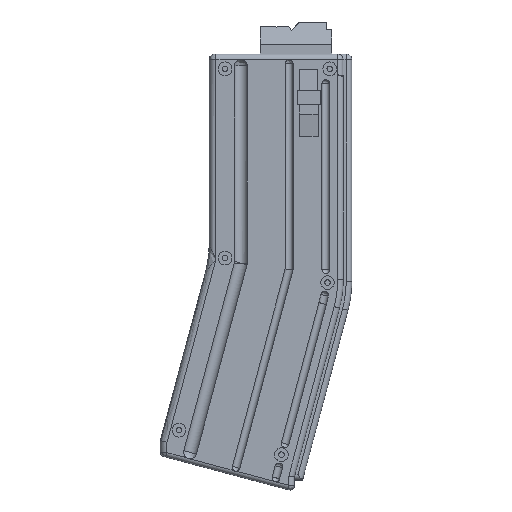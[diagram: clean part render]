
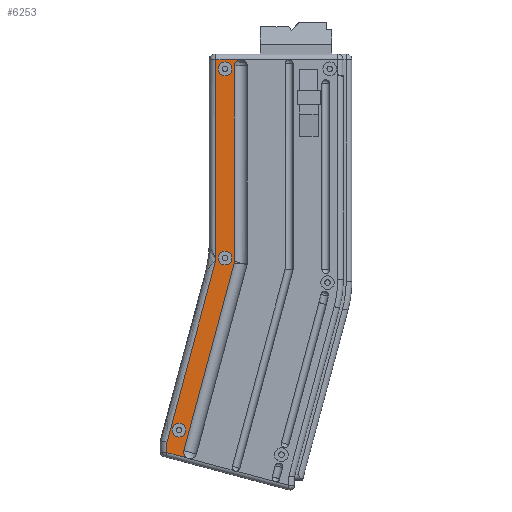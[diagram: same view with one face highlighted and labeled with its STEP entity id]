
A CAD part, front view. The second image highlights one B-rep face of the part: STEP entity #6253.
In plain terms, the highlighted planar face has unit normal (0, -1, 0).
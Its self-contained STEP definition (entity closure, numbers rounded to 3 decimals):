
#37=FACE_BOUND('',#1269,.T.);
#38=FACE_BOUND('',#1270,.T.);
#39=FACE_BOUND('',#1271,.T.);
#191=B_SPLINE_CURVE_WITH_KNOTS('',3,(#9843,#9844,#9845,#9846,#9847,#9848,
#9849,#9850,#9851,#9852,#9853,#9854),.UNSPECIFIED.,.F.,.F.,(4,2,2,2,2,4),
(0.,0.112,0.224,0.335,0.439,
0.44),.UNSPECIFIED.);
#193=B_SPLINE_CURVE_WITH_KNOTS('',3,(#9987,#9988,#9989,#9990,#9991,#9992,
#9993,#9994,#9995,#9996,#9997,#9998),.UNSPECIFIED.,.F.,.F.,(4,2,2,2,2,4),
(-0.001,0.,0.105,0.216,0.327,
0.439),.UNSPECIFIED.);
#195=B_SPLINE_CURVE_WITH_KNOTS('',3,(#10056,#10057,#10058,#10059,#10060,
#10061,#10062,#10063,#10064,#10065,#10066,#10067,#10068),.UNSPECIFIED.,
 .F.,.F.,(4,3,3,3,4),(0.,0.024,0.037,0.061,
0.073),.UNSPECIFIED.);
#656=CIRCLE('',#6703,3.075);
#657=CIRCLE('',#6704,3.075);
#658=CIRCLE('',#6705,3.075);
#876=FACE_OUTER_BOUND('',#1268,.T.);
#1268=EDGE_LOOP('',(#4353,#4354,#4355,#4356,#4357,#4358,#4359,#4360,#4361,
#4362,#4363));
#1269=EDGE_LOOP('',(#4364));
#1270=EDGE_LOOP('',(#4365));
#1271=EDGE_LOOP('',(#4366));
#1661=LINE('',#9527,#2093);
#1685=LINE('',#9873,#2117);
#1687=LINE('',#10013,#2119);
#1688=LINE('',#10071,#2120);
#1689=LINE('',#10073,#2121);
#1690=LINE('',#10075,#2122);
#1691=LINE('',#10077,#2123);
#1692=LINE('',#10078,#2124);
#2093=VECTOR('',#7355,10.);
#2117=VECTOR('',#7413,10.);
#2119=VECTOR('',#7417,10.);
#2120=VECTOR('',#7424,10.);
#2121=VECTOR('',#7425,10.);
#2122=VECTOR('',#7426,10.);
#2123=VECTOR('',#7427,10.);
#2124=VECTOR('',#7428,10.);
#2559=VERTEX_POINT('',#9524);
#2560=VERTEX_POINT('',#9526);
#2594=VERTEX_POINT('',#9842);
#2596=VERTEX_POINT('',#9871);
#2597=VERTEX_POINT('',#9984);
#2598=VERTEX_POINT('',#9986);
#2599=VERTEX_POINT('',#10012);
#2600=VERTEX_POINT('',#10070);
#2601=VERTEX_POINT('',#10072);
#2602=VERTEX_POINT('',#10074);
#2603=VERTEX_POINT('',#10076);
#2604=VERTEX_POINT('',#10079);
#2605=VERTEX_POINT('',#10081);
#2606=VERTEX_POINT('',#10083);
#3208=EDGE_CURVE('',#2559,#2560,#1661,.T.);
#3249=EDGE_CURVE('',#2559,#2594,#191,.F.);
#3253=EDGE_CURVE('',#2594,#2596,#1685,.T.);
#3255=EDGE_CURVE('',#2597,#2598,#193,.T.);
#3257=EDGE_CURVE('',#2599,#2598,#1687,.T.);
#3260=EDGE_CURVE('',#2599,#2596,#195,.T.);
#3261=EDGE_CURVE('',#2600,#2597,#1688,.T.);
#3262=EDGE_CURVE('',#2601,#2600,#1689,.T.);
#3263=EDGE_CURVE('',#2601,#2602,#1690,.T.);
#3264=EDGE_CURVE('',#2603,#2602,#1691,.T.);
#3265=EDGE_CURVE('',#2560,#2603,#1692,.T.);
#3266=EDGE_CURVE('',#2604,#2604,#656,.T.);
#3267=EDGE_CURVE('',#2605,#2605,#657,.T.);
#3268=EDGE_CURVE('',#2606,#2606,#658,.T.);
#4353=ORIENTED_EDGE('',*,*,#3260,.F.);
#4354=ORIENTED_EDGE('',*,*,#3257,.T.);
#4355=ORIENTED_EDGE('',*,*,#3255,.F.);
#4356=ORIENTED_EDGE('',*,*,#3261,.F.);
#4357=ORIENTED_EDGE('',*,*,#3262,.F.);
#4358=ORIENTED_EDGE('',*,*,#3263,.T.);
#4359=ORIENTED_EDGE('',*,*,#3264,.F.);
#4360=ORIENTED_EDGE('',*,*,#3265,.F.);
#4361=ORIENTED_EDGE('',*,*,#3208,.F.);
#4362=ORIENTED_EDGE('',*,*,#3249,.T.);
#4363=ORIENTED_EDGE('',*,*,#3253,.T.);
#4364=ORIENTED_EDGE('',*,*,#3266,.T.);
#4365=ORIENTED_EDGE('',*,*,#3267,.T.);
#4366=ORIENTED_EDGE('',*,*,#3268,.T.);
#6064=PLANE('',#6702);
#6253=ADVANCED_FACE('',(#876,#37,#38,#39),#6064,.T.);
#6702=AXIS2_PLACEMENT_3D('',#10069,#7422,#7423);
#6703=AXIS2_PLACEMENT_3D('',#10080,#7429,#7430);
#6704=AXIS2_PLACEMENT_3D('',#10082,#7431,#7432);
#6705=AXIS2_PLACEMENT_3D('',#10084,#7433,#7434);
#7355=DIRECTION('',(-0.966,0.,0.259));
#7413=DIRECTION('',(0.259,0.,0.966));
#7417=DIRECTION('',(0.,0.,1.));
#7422=DIRECTION('center_axis',(0.,-1.,0.));
#7423=DIRECTION('ref_axis',(1.,0.,0.));
#7424=DIRECTION('',(1.,0.,0.));
#7425=DIRECTION('',(0.,0.,1.));
#7426=DIRECTION('',(-0.259,0.,-0.966));
#7427=DIRECTION('',(0.966,0.,-0.259));
#7428=DIRECTION('',(0.,0.,1.));
#7429=DIRECTION('center_axis',(0.,1.,0.));
#7430=DIRECTION('ref_axis',(1.,0.,0.));
#7431=DIRECTION('center_axis',(0.,1.,0.));
#7432=DIRECTION('ref_axis',(1.,0.,0.));
#7433=DIRECTION('center_axis',(0.,1.,0.));
#7434=DIRECTION('ref_axis',(1.,0.,0.));
#9524=CARTESIAN_POINT('',(326.692,-38.877,-148.043));
#9526=CARTESIAN_POINT('',(317.124,-38.877,-145.479));
#9527=CARTESIAN_POINT('',(332.652,-38.877,-149.64));
#9842=CARTESIAN_POINT('',(324.724,-38.877,-144.621));
#9843=CARTESIAN_POINT('Ctrl Pts',(324.724,-38.877,-144.621));
#9844=CARTESIAN_POINT('Ctrl Pts',(324.627,-38.877,-144.982));
#9845=CARTESIAN_POINT('Ctrl Pts',(324.603,-38.877,-145.36));
#9846=CARTESIAN_POINT('Ctrl Pts',(324.705,-38.877,-146.098));
#9847=CARTESIAN_POINT('Ctrl Pts',(324.829,-38.877,-146.452));
#9848=CARTESIAN_POINT('Ctrl Pts',(325.206,-38.877,-147.09));
#9849=CARTESIAN_POINT('Ctrl Pts',(325.456,-38.877,-147.367));
#9850=CARTESIAN_POINT('Ctrl Pts',(326.033,-38.877,-147.796));
#9851=CARTESIAN_POINT('Ctrl Pts',(326.349,-38.877,-147.95));
#9852=CARTESIAN_POINT('Ctrl Pts',(326.688,-38.877,-148.041));
#9853=CARTESIAN_POINT('Ctrl Pts',(326.69,-38.877,-148.042));
#9854=CARTESIAN_POINT('Ctrl Pts',(326.692,-38.877,-148.043));
#9871=CARTESIAN_POINT('',(347.308,-38.877,-60.335));
#9873=CARTESIAN_POINT('',(324.,-38.877,-147.321));
#9984=CARTESIAN_POINT('',(350.191,-38.877,30.987));
#9986=CARTESIAN_POINT('',(347.403,-38.877,28.191));
#9987=CARTESIAN_POINT('Ctrl Pts',(350.191,-38.877,30.987));
#9988=CARTESIAN_POINT('Ctrl Pts',(350.188,-38.877,30.987));
#9989=CARTESIAN_POINT('Ctrl Pts',(350.186,-38.877,30.987));
#9990=CARTESIAN_POINT('Ctrl Pts',(349.835,-38.877,30.986));
#9991=CARTESIAN_POINT('Ctrl Pts',(349.49,-38.877,30.919));
#9992=CARTESIAN_POINT('Ctrl Pts',(348.822,-38.877,30.654));
#9993=CARTESIAN_POINT('Ctrl Pts',(348.508,-38.877,30.451));
#9994=CARTESIAN_POINT('Ctrl Pts',(347.979,-38.877,29.933));
#9995=CARTESIAN_POINT('Ctrl Pts',(347.768,-38.877,29.623));
#9996=CARTESIAN_POINT('Ctrl Pts',(347.478,-38.877,28.936));
#9997=CARTESIAN_POINT('Ctrl Pts',(347.403,-38.877,28.565));
#9998=CARTESIAN_POINT('Ctrl Pts',(347.403,-38.877,28.191));
#10012=CARTESIAN_POINT('',(347.403,-38.877,-59.611));
#10013=CARTESIAN_POINT('',(347.403,-38.877,-60.362));
#10056=CARTESIAN_POINT('Ctrl Pts',(347.403,-38.877,-59.611));
#10057=CARTESIAN_POINT('Ctrl Pts',(347.403,-38.877,-59.692));
#10058=CARTESIAN_POINT('Ctrl Pts',(347.4,-38.877,-59.773));
#10059=CARTESIAN_POINT('Ctrl Pts',(347.393,-38.877,-59.853));
#10060=CARTESIAN_POINT('Ctrl Pts',(347.389,-38.877,-59.894));
#10061=CARTESIAN_POINT('Ctrl Pts',(347.385,-38.877,-59.935));
#10062=CARTESIAN_POINT('Ctrl Pts',(347.379,-38.877,-59.976));
#10063=CARTESIAN_POINT('Ctrl Pts',(347.369,-38.877,-60.056));
#10064=CARTESIAN_POINT('Ctrl Pts',(347.355,-38.877,-60.136));
#10065=CARTESIAN_POINT('Ctrl Pts',(347.337,-38.877,-60.215));
#10066=CARTESIAN_POINT('Ctrl Pts',(347.329,-38.877,-60.255));
#10067=CARTESIAN_POINT('Ctrl Pts',(347.319,-38.877,-60.295));
#10068=CARTESIAN_POINT('Ctrl Pts',(347.308,-38.877,-60.335));
#10069=CARTESIAN_POINT('Origin',(356.451,-38.877,-60.928));
#10070=CARTESIAN_POINT('',(339.124,-38.877,30.987));
#10071=CARTESIAN_POINT('',(372.807,-38.877,30.987));
#10072=CARTESIAN_POINT('',(339.124,-38.877,-58.889));
#10073=CARTESIAN_POINT('',(339.124,-38.877,-60.891));
#10074=CARTESIAN_POINT('',(317.15,-38.877,-140.896));
#10075=CARTESIAN_POINT('',(339.124,-38.877,-58.889));
#10076=CARTESIAN_POINT('',(317.124,-38.877,-140.889));
#10077=CARTESIAN_POINT('',(337.867,-38.877,-146.447));
#10078=CARTESIAN_POINT('',(317.124,-38.877,-142.891));
#10079=CARTESIAN_POINT('',(340.168,-38.877,-58.134));
#10080=CARTESIAN_POINT('Origin',(343.243,-38.877,-58.134));
#10081=CARTESIAN_POINT('',(340.168,-38.877,26.866));
#10082=CARTESIAN_POINT('Origin',(343.243,-38.877,26.866));
#10083=CARTESIAN_POINT('',(319.462,-38.877,-135.408));
#10084=CARTESIAN_POINT('Origin',(322.537,-38.877,-135.408));
